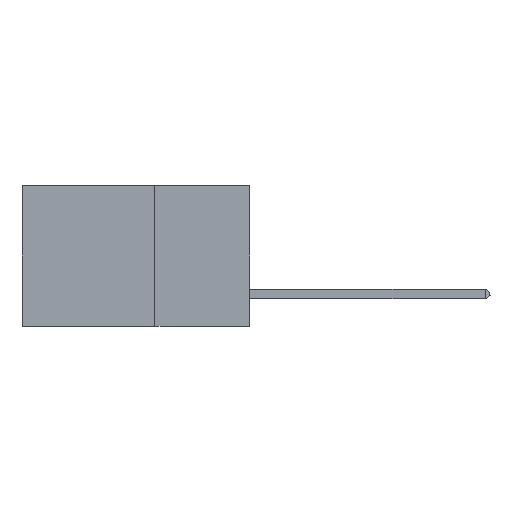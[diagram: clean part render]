
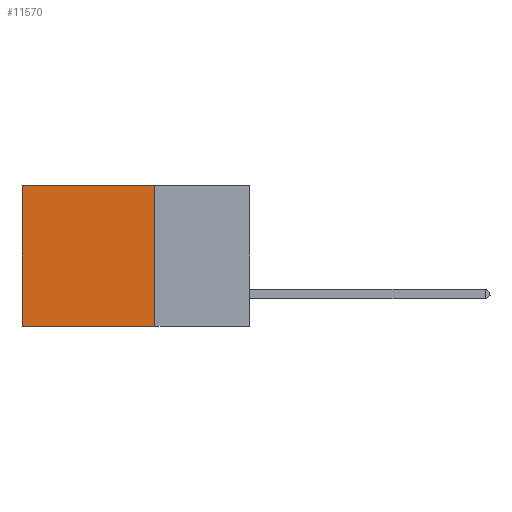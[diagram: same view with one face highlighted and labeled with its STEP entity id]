
A CAD part, left-side view. The second image highlights one B-rep face of the part: STEP entity #11570.
In plain terms, the highlighted planar face has unit normal (-1, 0, 0).
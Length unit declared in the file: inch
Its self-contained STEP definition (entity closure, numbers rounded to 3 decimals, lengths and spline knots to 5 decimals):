
#220 = EDGE_CURVE ( 'NONE', #11720, #19044, #11434, .T. ) ;
#2617 = VECTOR ( 'NONE', #11814, 39.37008 ) ;
#2733 = CARTESIAN_POINT ( 'NONE',  ( 0.2875, 0.6, 0. ) ) ;
#2914 = DIRECTION ( 'NONE',  ( 0., 0., -1. ) ) ;
#3171 = AXIS2_PLACEMENT_3D ( 'NONE', #8839, #23195, #10904 ) ;
#4413 = VECTOR ( 'NONE', #2914, 39.37008 ) ;
#4864 = EDGE_LOOP ( 'NONE', ( #20532, #5054, #11381, #19249 ) ) ;
#5054 = ORIENTED_EDGE ( 'NONE', *, *, #220, .F. ) ;
#5254 = VECTOR ( 'NONE', #24852, 39.37008 ) ;
#5576 = LINE ( 'NONE', #22371, #5254 ) ;
#7207 = EDGE_CURVE ( 'NONE', #10237, #19044, #25928, .T. ) ;
#7776 = LINE ( 'NONE', #11177, #2617 ) ;
#8839 = CARTESIAN_POINT ( 'NONE',  ( 0.2875, 0.25, 0. ) ) ;
#10237 = VERTEX_POINT ( 'NONE', #25247 ) ;
#10904 = DIRECTION ( 'NONE',  ( 0., 0., -1. ) ) ;
#10985 = PLANE ( 'NONE',  #3171 ) ;
#11177 = CARTESIAN_POINT ( 'NONE',  ( 0.2875, 0.25, 0. ) ) ;
#11381 = ORIENTED_EDGE ( 'NONE', *, *, #26197, .F. ) ;
#11434 = LINE ( 'NONE', #16142, #12747 ) ;
#11570 = ADVANCED_FACE ( 'NONE', ( #22944 ), #10985, .F. ) ;
#11720 = VERTEX_POINT ( 'NONE', #18008 ) ;
#11814 = DIRECTION ( 'NONE',  ( 0., 0., -1. ) ) ;
#12747 = VECTOR ( 'NONE', #13717, 39.37008 ) ;
#13717 = DIRECTION ( 'NONE',  ( 0., 1., 0. ) ) ;
#13740 = VERTEX_POINT ( 'NONE', #18986 ) ;
#16142 = CARTESIAN_POINT ( 'NONE',  ( 0.2875, 0.25, -0.37 ) ) ;
#18008 = CARTESIAN_POINT ( 'NONE',  ( 0.2875, 0.25, -0.37 ) ) ;
#18637 = CARTESIAN_POINT ( 'NONE',  ( 0.2875, 0.6, -0.37 ) ) ;
#18986 = CARTESIAN_POINT ( 'NONE',  ( 0.2875, 0.25, 0. ) ) ;
#19044 = VERTEX_POINT ( 'NONE', #18637 ) ;
#19249 = ORIENTED_EDGE ( 'NONE', *, *, #22488, .T. ) ;
#20532 = ORIENTED_EDGE ( 'NONE', *, *, #7207, .T. ) ;
#22371 = CARTESIAN_POINT ( 'NONE',  ( 0.2875, 0.25, 0. ) ) ;
#22488 = EDGE_CURVE ( 'NONE', #13740, #10237, #5576, .T. ) ;
#22944 = FACE_OUTER_BOUND ( 'NONE', #4864, .T. ) ;
#23195 = DIRECTION ( 'NONE',  ( 1., 0., 0. ) ) ;
#24852 = DIRECTION ( 'NONE',  ( 0., 1., 0. ) ) ;
#25247 = CARTESIAN_POINT ( 'NONE',  ( 0.2875, 0.6, 0. ) ) ;
#25928 = LINE ( 'NONE', #2733, #4413 ) ;
#26197 = EDGE_CURVE ( 'NONE', #13740, #11720, #7776, .T. ) ;
